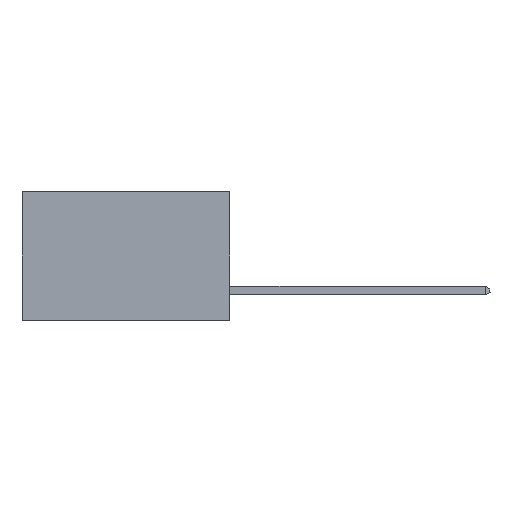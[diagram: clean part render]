
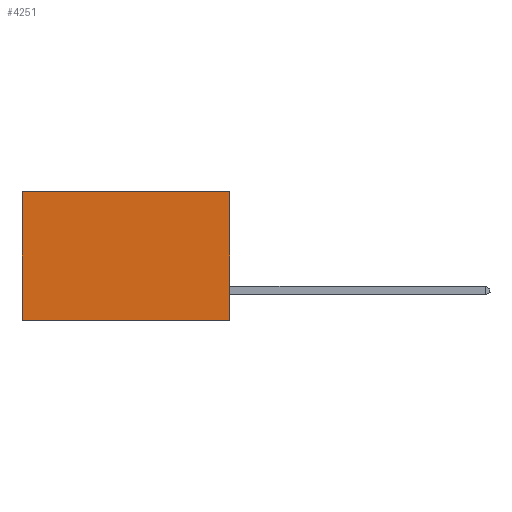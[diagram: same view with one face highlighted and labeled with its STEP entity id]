
A CAD part, left-side view. The second image highlights one B-rep face of the part: STEP entity #4251.
In plain terms, the highlighted planar face has unit normal (-1, 0, 0).
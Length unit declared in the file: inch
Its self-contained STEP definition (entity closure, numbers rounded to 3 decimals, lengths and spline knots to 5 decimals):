
#369 = DIRECTION ( 'NONE',  ( 1., 0., 0. ) ) ;
#372 = ORIENTED_EDGE ( 'NONE', *, *, #8390, .F. ) ;
#719 = LINE ( 'NONE', #7682, #5281 ) ;
#1009 = ORIENTED_EDGE ( 'NONE', *, *, #4854, .T. ) ;
#1044 = VERTEX_POINT ( 'NONE', #1818 ) ;
#1223 = ORIENTED_EDGE ( 'NONE', *, *, #8291, .T. ) ;
#1344 = EDGE_CURVE ( 'NONE', #1044, #4062, #719, .T. ) ;
#1530 = CARTESIAN_POINT ( 'NONE',  ( 0.298, 0.6, -0.37 ) ) ;
#1573 = LINE ( 'NONE', #5543, #2641 ) ;
#1818 = CARTESIAN_POINT ( 'NONE',  ( 0.298, 0., 0. ) ) ;
#1870 = VERTEX_POINT ( 'NONE', #4683 ) ;
#1882 = CARTESIAN_POINT ( 'NONE',  ( 0.298, 0., -0.37 ) ) ;
#1945 = LINE ( 'NONE', #1882, #5918 ) ;
#2115 = ORIENTED_EDGE ( 'NONE', *, *, #1344, .F. ) ;
#2259 = DIRECTION ( 'NONE',  ( 0., 0., -1. ) ) ;
#2641 = VECTOR ( 'NONE', #4178, 39.37008 ) ;
#2945 = EDGE_LOOP ( 'NONE', ( #1009, #372, #2115, #1223 ) ) ;
#3935 = LINE ( 'NONE', #7068, #8040 ) ;
#4062 = VERTEX_POINT ( 'NONE', #5266 ) ;
#4178 = DIRECTION ( 'NONE',  ( 0., 0., -1. ) ) ;
#4251 = ADVANCED_FACE ( 'NONE', ( #7874 ), #8320, .F. ) ;
#4386 = DIRECTION ( 'NONE',  ( 0., 1., 0. ) ) ;
#4683 = CARTESIAN_POINT ( 'NONE',  ( 0.298, 0.6, 0. ) ) ;
#4854 = EDGE_CURVE ( 'NONE', #1870, #8103, #1573, .T. ) ;
#5117 = DIRECTION ( 'NONE',  ( 0., 1., 0. ) ) ;
#5266 = CARTESIAN_POINT ( 'NONE',  ( 0.298, 0., -0.37 ) ) ;
#5281 = VECTOR ( 'NONE', #2259, 39.37008 ) ;
#5477 = AXIS2_PLACEMENT_3D ( 'NONE', #6312, #369, #5712 ) ;
#5543 = CARTESIAN_POINT ( 'NONE',  ( 0.298, 0.6, 0. ) ) ;
#5712 = DIRECTION ( 'NONE',  ( 0., 0., -1. ) ) ;
#5918 = VECTOR ( 'NONE', #5117, 39.37008 ) ;
#6312 = CARTESIAN_POINT ( 'NONE',  ( 0.298, 0., 0. ) ) ;
#7068 = CARTESIAN_POINT ( 'NONE',  ( 0.298, 0., 0. ) ) ;
#7682 = CARTESIAN_POINT ( 'NONE',  ( 0.298, 0., 0. ) ) ;
#7874 = FACE_OUTER_BOUND ( 'NONE', #2945, .T. ) ;
#8040 = VECTOR ( 'NONE', #4386, 39.37008 ) ;
#8103 = VERTEX_POINT ( 'NONE', #1530 ) ;
#8291 = EDGE_CURVE ( 'NONE', #1044, #1870, #3935, .T. ) ;
#8320 = PLANE ( 'NONE',  #5477 ) ;
#8390 = EDGE_CURVE ( 'NONE', #4062, #8103, #1945, .T. ) ;
